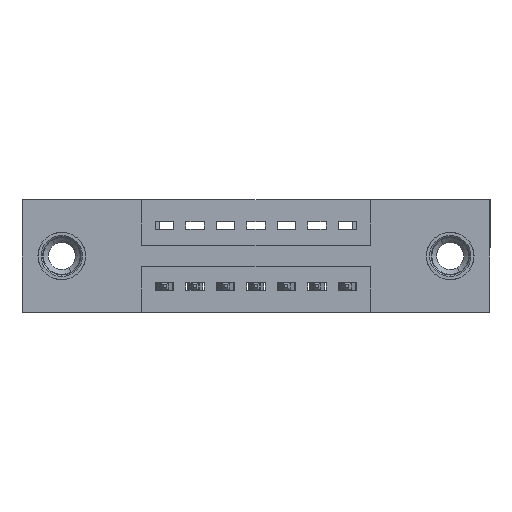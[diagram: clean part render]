
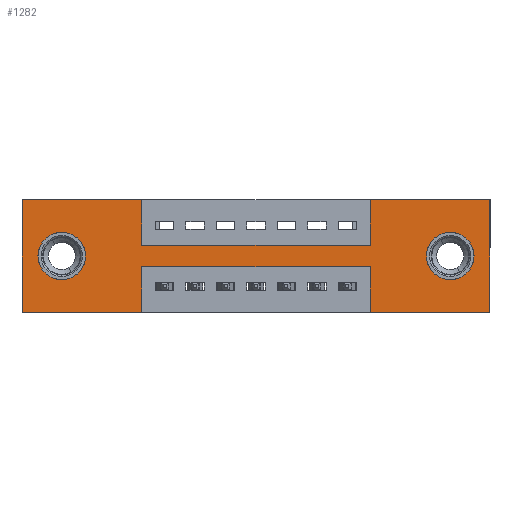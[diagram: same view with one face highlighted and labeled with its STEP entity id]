
A CAD part, front view. The second image highlights one B-rep face of the part: STEP entity #1282.
In plain terms, the highlighted planar face has unit normal (0, -1, 0).
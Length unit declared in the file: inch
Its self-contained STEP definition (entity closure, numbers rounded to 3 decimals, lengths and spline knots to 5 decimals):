
#50 = VECTOR ( 'NONE', #1359, 39.37008 ) ;
#346 = EDGE_CURVE ( 'NONE', #3852, #8562, #11605, .T. ) ;
#428 = CARTESIAN_POINT ( 'NONE',  ( 0., 0., -0.37 ) ) ;
#575 = DIRECTION ( 'NONE',  ( 0., 0., -1. ) ) ;
#580 = LINE ( 'NONE', #720, #6257 ) ;
#720 = CARTESIAN_POINT ( 'NONE',  ( 0., 0., 0. ) ) ;
#811 = VERTEX_POINT ( 'NONE', #1590 ) ;
#836 = CARTESIAN_POINT ( 'NONE',  ( 0.13, 0., -0.107 ) ) ;
#862 = VECTOR ( 'NONE', #13215, 39.37008 ) ;
#1014 = VERTEX_POINT ( 'NONE', #12106 ) ;
#1136 = EDGE_CURVE ( 'NONE', #11665, #4611, #7064, .T. ) ;
#1282 = ADVANCED_FACE ( 'NONE', ( #13874, #4745, #6688 ), #7752, .T. ) ;
#1359 = DIRECTION ( 'NONE',  ( 0., 0., -1. ) ) ;
#1467 = LINE ( 'NONE', #6100, #3794 ) ;
#1562 = VERTEX_POINT ( 'NONE', #6940 ) ;
#1590 = CARTESIAN_POINT ( 'NONE',  ( 0., 0., -0.37 ) ) ;
#1691 = LINE ( 'NONE', #3914, #7779 ) ;
#2106 = CARTESIAN_POINT ( 'NONE',  ( 0.3925, 0., 0. ) ) ;
#2253 = VERTEX_POINT ( 'NONE', #2870 ) ;
#2389 = ORIENTED_EDGE ( 'NONE', *, *, #4139, .F. ) ;
#2401 = ORIENTED_EDGE ( 'NONE', *, *, #6496, .F. ) ;
#2436 = VECTOR ( 'NONE', #12427, 39.37008 ) ;
#2870 = CARTESIAN_POINT ( 'NONE',  ( 0.3925, 0., -0.15 ) ) ;
#3043 = CARTESIAN_POINT ( 'NONE',  ( 1.405, 0., -0.185 ) ) ;
#3095 = DIRECTION ( 'NONE',  ( 0., 0., -1. ) ) ;
#3156 = DIRECTION ( 'NONE',  ( 0., 1., 0. ) ) ;
#3175 = CARTESIAN_POINT ( 'NONE',  ( 1.1425, 0., 0. ) ) ;
#3444 = LINE ( 'NONE', #9376, #50 ) ;
#3673 = ORIENTED_EDGE ( 'NONE', *, *, #12744, .F. ) ;
#3794 = VECTOR ( 'NONE', #4907, 39.37008 ) ;
#3827 = CARTESIAN_POINT ( 'NONE',  ( 1.405, 0., -0.263 ) ) ;
#3852 = VERTEX_POINT ( 'NONE', #4804 ) ;
#3870 = ORIENTED_EDGE ( 'NONE', *, *, #7519, .T. ) ;
#3891 = CARTESIAN_POINT ( 'NONE',  ( 0.3925, 0., -0.37 ) ) ;
#3914 = CARTESIAN_POINT ( 'NONE',  ( 0.3925, 0., -0.15 ) ) ;
#4139 = EDGE_CURVE ( 'NONE', #8562, #7398, #10261, .T. ) ;
#4156 = AXIS2_PLACEMENT_3D ( 'NONE', #14663, #7633, #8811 ) ;
#4546 = AXIS2_PLACEMENT_3D ( 'NONE', #8978, #14617, #7788 ) ;
#4611 = VERTEX_POINT ( 'NONE', #3891 ) ;
#4664 = CARTESIAN_POINT ( 'NONE',  ( 0., 0., -0.37 ) ) ;
#4702 = EDGE_CURVE ( 'NONE', #12298, #8567, #10417, .T. ) ;
#4745 = FACE_BOUND ( 'NONE', #13031, .T. ) ;
#4804 = CARTESIAN_POINT ( 'NONE',  ( 1.1425, 0., 0. ) ) ;
#4907 = DIRECTION ( 'NONE',  ( 0., 0., 1. ) ) ;
#5202 = VECTOR ( 'NONE', #8022, 39.37008 ) ;
#5288 = VECTOR ( 'NONE', #575, 39.37008 ) ;
#5333 = VERTEX_POINT ( 'NONE', #13557 ) ;
#5393 = DIRECTION ( 'NONE',  ( 0., 1., 0. ) ) ;
#5399 = ORIENTED_EDGE ( 'NONE', *, *, #10039, .F. ) ;
#5461 = LINE ( 'NONE', #9001, #2436 ) ;
#5728 = DIRECTION ( 'NONE',  ( 0., 0., -1. ) ) ;
#5787 = CIRCLE ( 'NONE', #14108, 0.078 ) ;
#5894 = EDGE_CURVE ( 'NONE', #1562, #11665, #5461, .T. ) ;
#5933 = CARTESIAN_POINT ( 'NONE',  ( 1.535, 0., 0. ) ) ;
#6087 = DIRECTION ( 'NONE',  ( 0., 0., 1. ) ) ;
#6100 = CARTESIAN_POINT ( 'NONE',  ( 1.1425, 0., -0.37 ) ) ;
#6117 = CARTESIAN_POINT ( 'NONE',  ( 0., 0., 0. ) ) ;
#6141 = ORIENTED_EDGE ( 'NONE', *, *, #12271, .F. ) ;
#6235 = CARTESIAN_POINT ( 'NONE',  ( 0.3925, 0., -0.37 ) ) ;
#6257 = VECTOR ( 'NONE', #9912, 39.37008 ) ;
#6496 = EDGE_CURVE ( 'NONE', #4611, #811, #9569, .T. ) ;
#6499 = EDGE_CURVE ( 'NONE', #8567, #12298, #12599, .T. ) ;
#6688 = FACE_OUTER_BOUND ( 'NONE', #12634, .T. ) ;
#6716 = DIRECTION ( 'NONE',  ( -1., 0., 0. ) ) ;
#6834 = DIRECTION ( 'NONE',  ( 0., -1., 0. ) ) ;
#6842 = ORIENTED_EDGE ( 'NONE', *, *, #346, .F. ) ;
#6940 = CARTESIAN_POINT ( 'NONE',  ( 1.1425, 0., -0.22 ) ) ;
#7064 = LINE ( 'NONE', #6235, #5288 ) ;
#7141 = ORIENTED_EDGE ( 'NONE', *, *, #5894, .F. ) ;
#7215 = VERTEX_POINT ( 'NONE', #6117 ) ;
#7319 = EDGE_LOOP ( 'NONE', ( #8270, #10133 ) ) ;
#7398 = VERTEX_POINT ( 'NONE', #9908 ) ;
#7519 = EDGE_CURVE ( 'NONE', #10715, #1014, #11698, .T. ) ;
#7633 = DIRECTION ( 'NONE',  ( 0., 1., 0. ) ) ;
#7752 = PLANE ( 'NONE',  #9967 ) ;
#7779 = VECTOR ( 'NONE', #8384, 39.37008 ) ;
#7788 = DIRECTION ( 'NONE',  ( 0., 0., -1. ) ) ;
#7845 = EDGE_CURVE ( 'NONE', #7215, #8366, #580, .T. ) ;
#8022 = DIRECTION ( 'NONE',  ( 0., 0., -1. ) ) ;
#8270 = ORIENTED_EDGE ( 'NONE', *, *, #6499, .T. ) ;
#8337 = EDGE_CURVE ( 'NONE', #1014, #10715, #5787, .T. ) ;
#8350 = CARTESIAN_POINT ( 'NONE',  ( 0.3925, 0., -0.22 ) ) ;
#8366 = VERTEX_POINT ( 'NONE', #2106 ) ;
#8384 = DIRECTION ( 'NONE',  ( 1., 0., 0. ) ) ;
#8410 = LINE ( 'NONE', #13941, #14104 ) ;
#8450 = LINE ( 'NONE', #428, #12383 ) ;
#8482 = EDGE_CURVE ( 'NONE', #7398, #11968, #8450, .T. ) ;
#8562 = VERTEX_POINT ( 'NONE', #11670 ) ;
#8567 = VERTEX_POINT ( 'NONE', #12873 ) ;
#8811 = DIRECTION ( 'NONE',  ( 0., 0., 1. ) ) ;
#8978 = CARTESIAN_POINT ( 'NONE',  ( 1.405, 0., -0.185 ) ) ;
#9001 = CARTESIAN_POINT ( 'NONE',  ( 0.3925, 0., -0.22 ) ) ;
#9070 = CARTESIAN_POINT ( 'NONE',  ( 1.1425, 0., -0.37 ) ) ;
#9131 = VECTOR ( 'NONE', #9442, 39.37008 ) ;
#9376 = CARTESIAN_POINT ( 'NONE',  ( 0.3925, 0., 0. ) ) ;
#9442 = DIRECTION ( 'NONE',  ( 0., 0., 1. ) ) ;
#9569 = LINE ( 'NONE', #10238, #12934 ) ;
#9908 = CARTESIAN_POINT ( 'NONE',  ( 1.535, 0., -0.37 ) ) ;
#9912 = DIRECTION ( 'NONE',  ( 1., 0., 0. ) ) ;
#9967 = AXIS2_PLACEMENT_3D ( 'NONE', #4664, #6834, #5728 ) ;
#9974 = DIRECTION ( 'NONE',  ( 0., 0., 1. ) ) ;
#9984 = ORIENTED_EDGE ( 'NONE', *, *, #13095, .F. ) ;
#10035 = CARTESIAN_POINT ( 'NONE',  ( 0.13, 0., -0.185 ) ) ;
#10039 = EDGE_CURVE ( 'NONE', #811, #7215, #8410, .T. ) ;
#10133 = ORIENTED_EDGE ( 'NONE', *, *, #4702, .T. ) ;
#10238 = CARTESIAN_POINT ( 'NONE',  ( 0., 0., -0.37 ) ) ;
#10261 = LINE ( 'NONE', #5933, #5202 ) ;
#10417 = CIRCLE ( 'NONE', #12928, 0.078 ) ;
#10459 = ORIENTED_EDGE ( 'NONE', *, *, #1136, .F. ) ;
#10470 = EDGE_CURVE ( 'NONE', #5333, #3852, #11795, .T. ) ;
#10643 = ORIENTED_EDGE ( 'NONE', *, *, #10470, .F. ) ;
#10715 = VERTEX_POINT ( 'NONE', #836 ) ;
#11605 = LINE ( 'NONE', #12034, #862 ) ;
#11665 = VERTEX_POINT ( 'NONE', #8350 ) ;
#11670 = CARTESIAN_POINT ( 'NONE',  ( 1.535, 0., 0. ) ) ;
#11698 = CIRCLE ( 'NONE', #4156, 0.078 ) ;
#11795 = LINE ( 'NONE', #3175, #9131 ) ;
#11961 = DIRECTION ( 'NONE',  ( -1., 0., 0. ) ) ;
#11968 = VERTEX_POINT ( 'NONE', #9070 ) ;
#12034 = CARTESIAN_POINT ( 'NONE',  ( 0., 0., 0. ) ) ;
#12106 = CARTESIAN_POINT ( 'NONE',  ( 0.13, 0., -0.263 ) ) ;
#12271 = EDGE_CURVE ( 'NONE', #2253, #5333, #1691, .T. ) ;
#12298 = VERTEX_POINT ( 'NONE', #3827 ) ;
#12354 = ORIENTED_EDGE ( 'NONE', *, *, #8482, .F. ) ;
#12383 = VECTOR ( 'NONE', #11961, 39.37008 ) ;
#12427 = DIRECTION ( 'NONE',  ( -1., 0., 0. ) ) ;
#12599 = CIRCLE ( 'NONE', #4546, 0.078 ) ;
#12634 = EDGE_LOOP ( 'NONE', ( #10459, #7141, #3673, #12354, #2389, #6842, #10643, #6141, #9984, #13379, #5399, #2401 ) ) ;
#12744 = EDGE_CURVE ( 'NONE', #11968, #1562, #1467, .T. ) ;
#12873 = CARTESIAN_POINT ( 'NONE',  ( 1.405, 0., -0.107 ) ) ;
#12928 = AXIS2_PLACEMENT_3D ( 'NONE', #3043, #5393, #3095 ) ;
#12934 = VECTOR ( 'NONE', #6716, 39.37008 ) ;
#13031 = EDGE_LOOP ( 'NONE', ( #3870, #13483 ) ) ;
#13095 = EDGE_CURVE ( 'NONE', #8366, #2253, #3444, .T. ) ;
#13215 = DIRECTION ( 'NONE',  ( 1., 0., 0. ) ) ;
#13379 = ORIENTED_EDGE ( 'NONE', *, *, #7845, .F. ) ;
#13483 = ORIENTED_EDGE ( 'NONE', *, *, #8337, .T. ) ;
#13557 = CARTESIAN_POINT ( 'NONE',  ( 1.1425, 0., -0.15 ) ) ;
#13874 = FACE_BOUND ( 'NONE', #7319, .T. ) ;
#13941 = CARTESIAN_POINT ( 'NONE',  ( 0., 0., 0. ) ) ;
#14104 = VECTOR ( 'NONE', #6087, 39.37008 ) ;
#14108 = AXIS2_PLACEMENT_3D ( 'NONE', #10035, #3156, #9974 ) ;
#14617 = DIRECTION ( 'NONE',  ( 0., 1., 0. ) ) ;
#14663 = CARTESIAN_POINT ( 'NONE',  ( 0.13, 0., -0.185 ) ) ;
